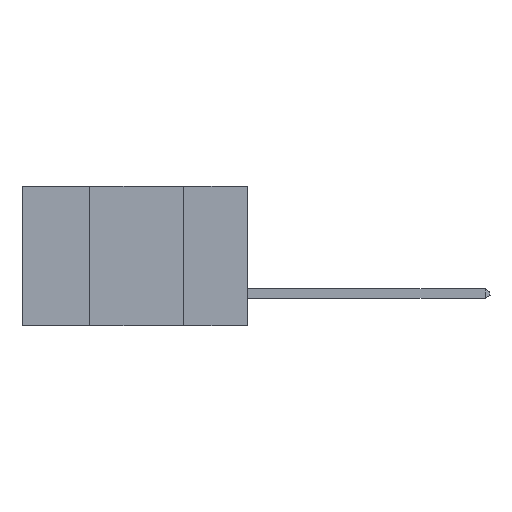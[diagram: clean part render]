
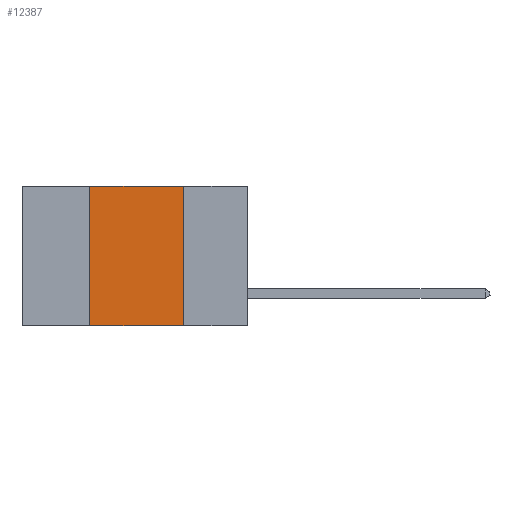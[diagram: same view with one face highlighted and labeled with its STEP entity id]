
A CAD part, left-side view. The second image highlights one B-rep face of the part: STEP entity #12387.
In plain terms, the highlighted planar face has unit normal (-1, 0, 0).
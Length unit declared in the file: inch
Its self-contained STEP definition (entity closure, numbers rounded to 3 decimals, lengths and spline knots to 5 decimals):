
#144 = CARTESIAN_POINT ( 'NONE',  ( 0., 0.6, -0.37 ) ) ;
#146 = LINE ( 'NONE', #1507, #14389 ) ;
#339 = ORIENTED_EDGE ( 'NONE', *, *, #1792, .F. ) ;
#513 = EDGE_LOOP ( 'NONE', ( #4233, #339, #5310, #5092 ) ) ;
#559 = CARTESIAN_POINT ( 'NONE',  ( 0., 0.17, 0. ) ) ;
#1184 = VECTOR ( 'NONE', #17344, 39.37008 ) ;
#1507 = CARTESIAN_POINT ( 'NONE',  ( 0., 0.17, 0. ) ) ;
#1792 = EDGE_CURVE ( 'NONE', #16896, #13856, #17013, .T. ) ;
#2390 = AXIS2_PLACEMENT_3D ( 'NONE', #16833, #12642, #16660 ) ;
#3762 = CARTESIAN_POINT ( 'NONE',  ( 0., 0.42, 0. ) ) ;
#4233 = ORIENTED_EDGE ( 'NONE', *, *, #17644, .F. ) ;
#4959 = VECTOR ( 'NONE', #5718, 39.37008 ) ;
#5024 = EDGE_CURVE ( 'NONE', #15442, #16896, #17686, .T. ) ;
#5092 = ORIENTED_EDGE ( 'NONE', *, *, #8376, .T. ) ;
#5282 = PLANE ( 'NONE',  #2390 ) ;
#5310 = ORIENTED_EDGE ( 'NONE', *, *, #5024, .F. ) ;
#5718 = DIRECTION ( 'NONE',  ( 0., -1., 0. ) ) ;
#5975 = VERTEX_POINT ( 'NONE', #9258 ) ;
#6021 = CARTESIAN_POINT ( 'NONE',  ( 0., 0.42, -0.37 ) ) ;
#8376 = EDGE_CURVE ( 'NONE', #15442, #5975, #9373, .T. ) ;
#8622 = CARTESIAN_POINT ( 'NONE',  ( 0., 0.6, 0. ) ) ;
#9258 = CARTESIAN_POINT ( 'NONE',  ( 0., 0.17, -0.37 ) ) ;
#9312 = VECTOR ( 'NONE', #10726, 39.37008 ) ;
#9373 = LINE ( 'NONE', #144, #1184 ) ;
#10726 = DIRECTION ( 'NONE',  ( 0., 0., 1. ) ) ;
#12387 = ADVANCED_FACE ( 'NONE', ( #13745 ), #5282, .F. ) ;
#12642 = DIRECTION ( 'NONE',  ( 1., 0., 0. ) ) ;
#13745 = FACE_OUTER_BOUND ( 'NONE', #513, .T. ) ;
#13856 = VERTEX_POINT ( 'NONE', #559 ) ;
#14301 = DIRECTION ( 'NONE',  ( 0., 0., -1. ) ) ;
#14389 = VECTOR ( 'NONE', #14301, 39.37008 ) ;
#14946 = CARTESIAN_POINT ( 'NONE',  ( 0., 0.42, 0. ) ) ;
#15442 = VERTEX_POINT ( 'NONE', #6021 ) ;
#16660 = DIRECTION ( 'NONE',  ( 0., 0., -1. ) ) ;
#16833 = CARTESIAN_POINT ( 'NONE',  ( 0., 0.6, 0. ) ) ;
#16896 = VERTEX_POINT ( 'NONE', #3762 ) ;
#17013 = LINE ( 'NONE', #8622, #4959 ) ;
#17344 = DIRECTION ( 'NONE',  ( 0., -1., 0. ) ) ;
#17644 = EDGE_CURVE ( 'NONE', #13856, #5975, #146, .T. ) ;
#17686 = LINE ( 'NONE', #14946, #9312 ) ;
